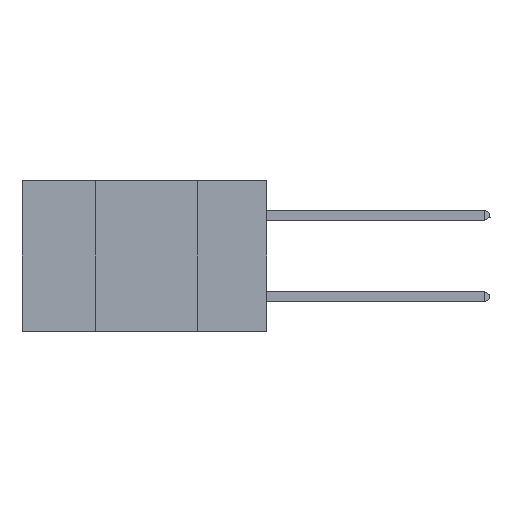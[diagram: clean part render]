
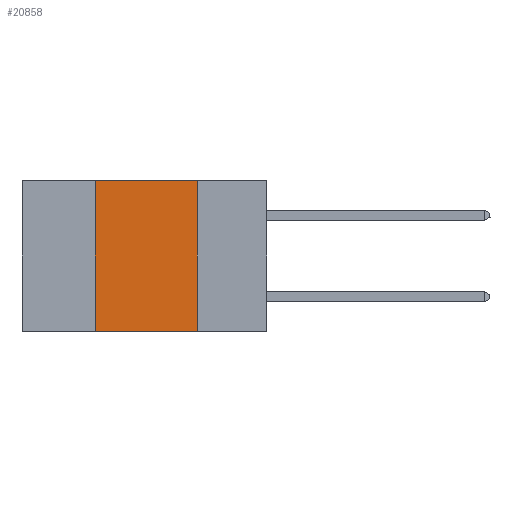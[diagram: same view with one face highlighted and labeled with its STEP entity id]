
A CAD part, left-side view. The second image highlights one B-rep face of the part: STEP entity #20858.
In plain terms, the highlighted planar face has unit normal (-1, 0, 0).
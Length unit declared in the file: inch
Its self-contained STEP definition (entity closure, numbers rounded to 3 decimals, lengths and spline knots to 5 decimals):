
#1834 = AXIS2_PLACEMENT_3D ( 'NONE', #37022, #19861, #30250 ) ;
#2002 = VERTEX_POINT ( 'NONE', #6099 ) ;
#4896 = DIRECTION ( 'NONE',  ( 0., -1., 0. ) ) ;
#6099 = CARTESIAN_POINT ( 'NONE',  ( 0., 0.42, -0.37 ) ) ;
#6328 = VECTOR ( 'NONE', #34686, 39.37008 ) ;
#7371 = CARTESIAN_POINT ( 'NONE',  ( 0., 0.17, 0. ) ) ;
#7593 = LINE ( 'NONE', #7371, #6328 ) ;
#9408 = CARTESIAN_POINT ( 'NONE',  ( 0., 0.6, -0.37 ) ) ;
#9776 = ORIENTED_EDGE ( 'NONE', *, *, #23356, .F. ) ;
#11367 = VECTOR ( 'NONE', #27450, 39.37008 ) ;
#11661 = LINE ( 'NONE', #32435, #28739 ) ;
#11875 = CARTESIAN_POINT ( 'NONE',  ( 0., 0.17, 0. ) ) ;
#13938 = EDGE_CURVE ( 'NONE', #16717, #26292, #7593, .T. ) ;
#16717 = VERTEX_POINT ( 'NONE', #11875 ) ;
#19149 = EDGE_LOOP ( 'NONE', ( #21202, #32146, #9776, #27791 ) ) ;
#19861 = DIRECTION ( 'NONE',  ( 1., 0., 0. ) ) ;
#20858 = ADVANCED_FACE ( 'NONE', ( #26393 ), #34072, .F. ) ;
#20907 = LINE ( 'NONE', #37828, #11367 ) ;
#21202 = ORIENTED_EDGE ( 'NONE', *, *, #13938, .F. ) ;
#23356 = EDGE_CURVE ( 'NONE', #2002, #30326, #20907, .T. ) ;
#26292 = VERTEX_POINT ( 'NONE', #29050 ) ;
#26393 = FACE_OUTER_BOUND ( 'NONE', #19149, .T. ) ;
#27424 = DIRECTION ( 'NONE',  ( 0., -1., 0. ) ) ;
#27450 = DIRECTION ( 'NONE',  ( 0., 0., 1. ) ) ;
#27791 = ORIENTED_EDGE ( 'NONE', *, *, #43675, .T. ) ;
#28739 = VECTOR ( 'NONE', #4896, 39.37008 ) ;
#29050 = CARTESIAN_POINT ( 'NONE',  ( 0., 0.17, -0.37 ) ) ;
#30250 = DIRECTION ( 'NONE',  ( 0., 0., -1. ) ) ;
#30326 = VERTEX_POINT ( 'NONE', #32240 ) ;
#30582 = LINE ( 'NONE', #9408, #35302 ) ;
#32146 = ORIENTED_EDGE ( 'NONE', *, *, #44115, .F. ) ;
#32240 = CARTESIAN_POINT ( 'NONE',  ( 0., 0.42, 0. ) ) ;
#32435 = CARTESIAN_POINT ( 'NONE',  ( 0., 0.6, 0. ) ) ;
#34072 = PLANE ( 'NONE',  #1834 ) ;
#34686 = DIRECTION ( 'NONE',  ( 0., 0., -1. ) ) ;
#35302 = VECTOR ( 'NONE', #27424, 39.37008 ) ;
#37022 = CARTESIAN_POINT ( 'NONE',  ( 0., 0.6, 0. ) ) ;
#37828 = CARTESIAN_POINT ( 'NONE',  ( 0., 0.42, 0. ) ) ;
#43675 = EDGE_CURVE ( 'NONE', #2002, #26292, #30582, .T. ) ;
#44115 = EDGE_CURVE ( 'NONE', #30326, #16717, #11661, .T. ) ;
